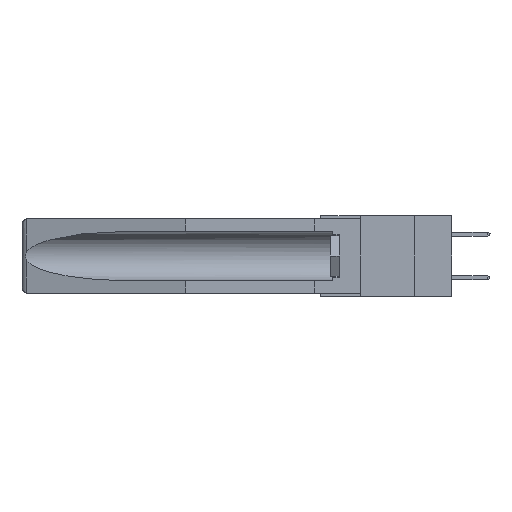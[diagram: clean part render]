
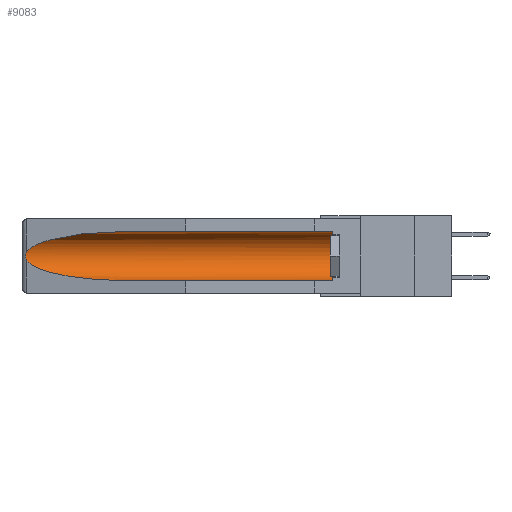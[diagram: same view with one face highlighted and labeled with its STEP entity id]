
A CAD part, left-side view. The second image highlights one B-rep face of the part: STEP entity #9083.
In plain terms, the highlighted cylindrical face has radius 2.857 mm (diameter 5.715 mm), a partial arc.
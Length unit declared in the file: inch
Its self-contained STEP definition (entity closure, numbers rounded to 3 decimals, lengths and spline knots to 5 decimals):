
#406 = VERTEX_POINT ( 'NONE', #12718 ) ;
#695 = CARTESIAN_POINT ( 'NONE',  ( 0.26537, 1.52718, -0.19328 ) ) ;
#1150 = DIRECTION ( 'NONE',  ( 0., 0., 1. ) ) ;
#1270 = AXIS2_PLACEMENT_3D ( 'NONE', #10887, #25177, #1150 ) ;
#2113 = AXIS2_PLACEMENT_3D ( 'NONE', #26046, #4126, #14239 ) ;
#2829 = LINE ( 'NONE', #22696, #4732 ) ;
#2842 = CIRCLE ( 'NONE', #1270, 0.1125 ) ;
#3491 = DIRECTION ( 'NONE',  ( 0., 1., 0. ) ) ;
#4126 = DIRECTION ( 'NONE',  ( 0., 1., 0. ) ) ;
#4732 = VECTOR ( 'NONE', #20452, 39.37008 ) ;
#5409 = CARTESIAN_POINT ( 'NONE',  ( 0.26654, 1.53092, -0.15636 ) ) ;
#5565 = CARTESIAN_POINT ( 'NONE',  ( 0.26537, 1.52718, -0.14972 ) ) ;
#5779 = B_SPLINE_CURVE_WITH_KNOTS ( 'NONE', 3,
 ( #5565, #21667, #5409, #19525, #9581, #21586, #23710, #17648, #11300, #21759 ),
 .UNSPECIFIED., .F., .F.,
 ( 4, 2, 2, 2, 4 ),
 ( 0., 0.00029, 0.00058, 0.00087, 0.00117 ),
 .UNSPECIFIED. ) ;
#6043 = VERTEX_POINT ( 'NONE', #19005 ) ;
#6401 = EDGE_CURVE ( 'NONE', #406, #13391, #7837, .T. ) ;
#6515 = ORIENTED_EDGE ( 'NONE', *, *, #14378, .F. ) ;
#7449 = EDGE_CURVE ( 'NONE', #24886, #16041, #2842, .T. ) ;
#7837 =( BOUNDED_CURVE ( )  B_SPLINE_CURVE ( 3, ( #25120, #18716, #16860, #18890 ),
 .UNSPECIFIED., .F., .F. ) 
 B_SPLINE_CURVE_WITH_KNOTS ( ( 4, 4 ),
 ( 4.71239, 6.08839 ),
 .UNSPECIFIED. ) 
 CURVE ( )  GEOMETRIC_REPRESENTATION_ITEM ( )  RATIONAL_B_SPLINE_CURVE ( ( 1., 0.848, 0.848, 1. ) ) 
 REPRESENTATION_ITEM ( '' )  );
#8764 = ORIENTED_EDGE ( 'NONE', *, *, #7449, .T. ) ;
#9083 = ADVANCED_FACE ( 'NONE', ( #22346 ), #23622, .F. ) ;
#9581 = CARTESIAN_POINT ( 'NONE',  ( 0.2675, 1.53308, -0.16763 ) ) ;
#10100 =( BOUNDED_CURVE ( )  B_SPLINE_CURVE ( 3, ( #15842, #25774, #21712, #25867 ),
 .UNSPECIFIED., .F., .T. ) 
 B_SPLINE_CURVE_WITH_KNOTS ( ( 4, 4 ),
 ( 0.1948, 1.5708 ),
 .UNSPECIFIED. ) 
 CURVE ( )  GEOMETRIC_REPRESENTATION_ITEM ( )  RATIONAL_B_SPLINE_CURVE ( ( 1., 0.848, 0.848, 1. ) ) 
 REPRESENTATION_ITEM ( '' )  );
#10887 = CARTESIAN_POINT ( 'NONE',  ( 0.155, 0.126, -0.1715 ) ) ;
#11300 = CARTESIAN_POINT ( 'NONE',  ( 0.26597, 1.5296, -0.19026 ) ) ;
#12718 = CARTESIAN_POINT ( 'NONE',  ( 0.155, 1.07973, -0.059 ) ) ;
#12775 = ORIENTED_EDGE ( 'NONE', *, *, #19465, .T. ) ;
#13391 = VERTEX_POINT ( 'NONE', #19031 ) ;
#13544 = EDGE_CURVE ( 'NONE', #16041, #406, #2829, .T. ) ;
#13983 = EDGE_CURVE ( 'NONE', #17875, #6043, #10100, .T. ) ;
#14118 = CARTESIAN_POINT ( 'NONE',  ( 0.155, 0.126, -0.284 ) ) ;
#14239 = DIRECTION ( 'NONE',  ( 0., 0., 1. ) ) ;
#14378 = EDGE_CURVE ( 'NONE', #24886, #6043, #21421, .T. ) ;
#15842 = CARTESIAN_POINT ( 'NONE',  ( 0.26537, 1.52718, -0.19328 ) ) ;
#15851 = ORIENTED_EDGE ( 'NONE', *, *, #6401, .T. ) ;
#16031 = VECTOR ( 'NONE', #3491, 39.37008 ) ;
#16041 = VERTEX_POINT ( 'NONE', #19416 ) ;
#16860 = CARTESIAN_POINT ( 'NONE',  ( 0.25451, 1.48313, -0.09465 ) ) ;
#17485 = CARTESIAN_POINT ( 'NONE',  ( 0.155, -0.30754, -0.284 ) ) ;
#17648 = CARTESIAN_POINT ( 'NONE',  ( 0.26655, 1.53094, -0.18657 ) ) ;
#17875 = VERTEX_POINT ( 'NONE', #695 ) ;
#18716 = CARTESIAN_POINT ( 'NONE',  ( 0.21114, 1.30732, -0.059 ) ) ;
#18890 = CARTESIAN_POINT ( 'NONE',  ( 0.26537, 1.52718, -0.14972 ) ) ;
#19005 = CARTESIAN_POINT ( 'NONE',  ( 0.155, 1.07973, -0.284 ) ) ;
#19031 = CARTESIAN_POINT ( 'NONE',  ( 0.26537, 1.52718, -0.14972 ) ) ;
#19416 = CARTESIAN_POINT ( 'NONE',  ( 0.155, 0.126, -0.059 ) ) ;
#19465 = EDGE_CURVE ( 'NONE', #13391, #17875, #5779, .T. ) ;
#19525 = CARTESIAN_POINT ( 'NONE',  ( 0.2673, 1.5327, -0.16383 ) ) ;
#20452 = DIRECTION ( 'NONE',  ( 0., 1., 0. ) ) ;
#21421 = LINE ( 'NONE', #17485, #16031 ) ;
#21586 = CARTESIAN_POINT ( 'NONE',  ( 0.2675, 1.53308, -0.17534 ) ) ;
#21667 = CARTESIAN_POINT ( 'NONE',  ( 0.26597, 1.52961, -0.15275 ) ) ;
#21712 = CARTESIAN_POINT ( 'NONE',  ( 0.21114, 1.30732, -0.284 ) ) ;
#21759 = CARTESIAN_POINT ( 'NONE',  ( 0.26537, 1.52718, -0.19328 ) ) ;
#22346 = FACE_OUTER_BOUND ( 'NONE', #23091, .T. ) ;
#22696 = CARTESIAN_POINT ( 'NONE',  ( 0.155, -0.30754, -0.059 ) ) ;
#22857 = ORIENTED_EDGE ( 'NONE', *, *, #13544, .T. ) ;
#23091 = EDGE_LOOP ( 'NONE', ( #15851, #12775, #25202, #6515, #8764, #22857 ) ) ;
#23622 = CYLINDRICAL_SURFACE ( 'NONE', #2113, 0.1125 ) ;
#23710 = CARTESIAN_POINT ( 'NONE',  ( 0.2673, 1.53269, -0.17917 ) ) ;
#24886 = VERTEX_POINT ( 'NONE', #14118 ) ;
#25120 = CARTESIAN_POINT ( 'NONE',  ( 0.155, 1.07973, -0.059 ) ) ;
#25177 = DIRECTION ( 'NONE',  ( 0., -1., 0. ) ) ;
#25202 = ORIENTED_EDGE ( 'NONE', *, *, #13983, .T. ) ;
#25774 = CARTESIAN_POINT ( 'NONE',  ( 0.25451, 1.48313, -0.24835 ) ) ;
#25867 = CARTESIAN_POINT ( 'NONE',  ( 0.155, 1.07973, -0.284 ) ) ;
#26046 = CARTESIAN_POINT ( 'NONE',  ( 0.155, -0.30754, -0.1715 ) ) ;
